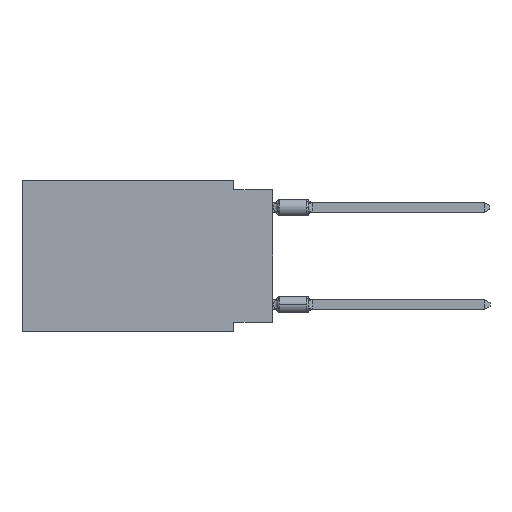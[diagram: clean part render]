
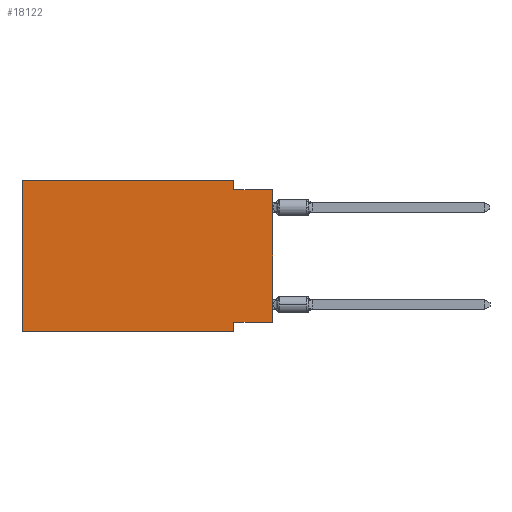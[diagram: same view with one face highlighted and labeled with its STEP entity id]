
A CAD part, left-side view. The second image highlights one B-rep face of the part: STEP entity #18122.
In plain terms, the highlighted planar face has unit normal (-1, 0, 0).
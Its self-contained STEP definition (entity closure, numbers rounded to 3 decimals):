
#65 = CARTESIAN_POINT ( 'NONE',  ( 0., 2.54, -0.635 ) ) ;
#612 = DIRECTION ( 'NONE',  ( 0., 0., -1. ) ) ;
#2394 = EDGE_CURVE ( 'NONE', #5224, #9709, #17510, .T. ) ;
#2664 = CARTESIAN_POINT ( 'NONE',  ( 0., 16.383, 0. ) ) ;
#2899 = LINE ( 'NONE', #14816, #19051 ) ;
#3383 = EDGE_CURVE ( 'NONE', #9709, #21280, #4348, .T. ) ;
#3583 = EDGE_CURVE ( 'NONE', #15294, #17643, #20864, .T. ) ;
#3847 = LINE ( 'NONE', #5370, #11055 ) ;
#4281 = ORIENTED_EDGE ( 'NONE', *, *, #8533, .F. ) ;
#4348 = LINE ( 'NONE', #7630, #15866 ) ;
#4852 = VERTEX_POINT ( 'NONE', #7908 ) ;
#4890 = VECTOR ( 'NONE', #11777, 1000. ) ;
#5224 = VERTEX_POINT ( 'NONE', #11243 ) ;
#5370 = CARTESIAN_POINT ( 'NONE',  ( 0., 2.54, -9.906 ) ) ;
#5894 = VERTEX_POINT ( 'NONE', #10645 ) ;
#6343 = DIRECTION ( 'NONE',  ( 0., 0., 1. ) ) ;
#6412 = FACE_OUTER_BOUND ( 'NONE', #13930, .T. ) ;
#6515 = DIRECTION ( 'NONE',  ( 1., 0., 0. ) ) ;
#7630 = CARTESIAN_POINT ( 'NONE',  ( 0., 2.54, 0. ) ) ;
#7699 = CARTESIAN_POINT ( 'NONE',  ( 0., 0., -9.271 ) ) ;
#7908 = CARTESIAN_POINT ( 'NONE',  ( 0., 16.383, -9.906 ) ) ;
#7989 = EDGE_CURVE ( 'NONE', #4852, #5894, #2899, .T. ) ;
#8114 = CARTESIAN_POINT ( 'NONE',  ( 0., 0., -9.271 ) ) ;
#8146 = PLANE ( 'NONE',  #20021 ) ;
#8533 = EDGE_CURVE ( 'NONE', #4852, #5224, #20075, .T. ) ;
#8867 = EDGE_CURVE ( 'NONE', #15294, #16092, #14559, .T. ) ;
#9025 = ORIENTED_EDGE ( 'NONE', *, *, #2394, .F. ) ;
#9709 = VERTEX_POINT ( 'NONE', #11443 ) ;
#10146 = CARTESIAN_POINT ( 'NONE',  ( 0., 16.383, 0. ) ) ;
#10645 = CARTESIAN_POINT ( 'NONE',  ( 0., 2.54, -9.906 ) ) ;
#11003 = EDGE_CURVE ( 'NONE', #17643, #5894, #3847, .T. ) ;
#11051 = DIRECTION ( 'NONE',  ( 0., 1., 0. ) ) ;
#11055 = VECTOR ( 'NONE', #612, 1000. ) ;
#11066 = VECTOR ( 'NONE', #13015, 1000. ) ;
#11243 = CARTESIAN_POINT ( 'NONE',  ( 0., 16.383, 0. ) ) ;
#11443 = CARTESIAN_POINT ( 'NONE',  ( 0., 2.54, 0. ) ) ;
#11448 = ORIENTED_EDGE ( 'NONE', *, *, #18036, .F. ) ;
#11509 = ORIENTED_EDGE ( 'NONE', *, *, #7989, .T. ) ;
#11777 = DIRECTION ( 'NONE',  ( 0., 0., 1. ) ) ;
#12785 = DIRECTION ( 'NONE',  ( 0., -1., 0. ) ) ;
#13015 = DIRECTION ( 'NONE',  ( 0., -1., 0. ) ) ;
#13034 = CARTESIAN_POINT ( 'NONE',  ( 0., 2.54, -9.271 ) ) ;
#13718 = ORIENTED_EDGE ( 'NONE', *, *, #8867, .T. ) ;
#13930 = EDGE_LOOP ( 'NONE', ( #13718, #11448, #20190, #9025, #4281, #11509, #19298, #15625 ) ) ;
#14559 = LINE ( 'NONE', #21149, #20101 ) ;
#14816 = CARTESIAN_POINT ( 'NONE',  ( 0., 16.383, -9.906 ) ) ;
#15294 = VERTEX_POINT ( 'NONE', #7699 ) ;
#15625 = ORIENTED_EDGE ( 'NONE', *, *, #3583, .F. ) ;
#15866 = VECTOR ( 'NONE', #20809, 1000. ) ;
#15908 = DIRECTION ( 'NONE',  ( 0., -1., 0. ) ) ;
#16092 = VERTEX_POINT ( 'NONE', #19101 ) ;
#16110 = VECTOR ( 'NONE', #15908, 1000. ) ;
#16373 = LINE ( 'NONE', #21220, #11066 ) ;
#17510 = LINE ( 'NONE', #2664, #16110 ) ;
#17643 = VERTEX_POINT ( 'NONE', #13034 ) ;
#17923 = VECTOR ( 'NONE', #11051, 1000. ) ;
#18036 = EDGE_CURVE ( 'NONE', #21280, #16092, #16373, .T. ) ;
#18122 = ADVANCED_FACE ( 'NONE', ( #6412 ), #8146, .F. ) ;
#19051 = VECTOR ( 'NONE', #12785, 1000. ) ;
#19101 = CARTESIAN_POINT ( 'NONE',  ( 0., 0., -0.635 ) ) ;
#19298 = ORIENTED_EDGE ( 'NONE', *, *, #11003, .F. ) ;
#19715 = DIRECTION ( 'NONE',  ( 0., 0., -1. ) ) ;
#20021 = AXIS2_PLACEMENT_3D ( 'NONE', #21324, #6515, #19715 ) ;
#20075 = LINE ( 'NONE', #10146, #4890 ) ;
#20101 = VECTOR ( 'NONE', #6343, 1000. ) ;
#20190 = ORIENTED_EDGE ( 'NONE', *, *, #3383, .F. ) ;
#20809 = DIRECTION ( 'NONE',  ( 0., 0., -1. ) ) ;
#20864 = LINE ( 'NONE', #8114, #17923 ) ;
#21149 = CARTESIAN_POINT ( 'NONE',  ( 0., 0., 0. ) ) ;
#21220 = CARTESIAN_POINT ( 'NONE',  ( 0., 0., -0.635 ) ) ;
#21280 = VERTEX_POINT ( 'NONE', #65 ) ;
#21324 = CARTESIAN_POINT ( 'NONE',  ( 0., 16.383, 0. ) ) ;
